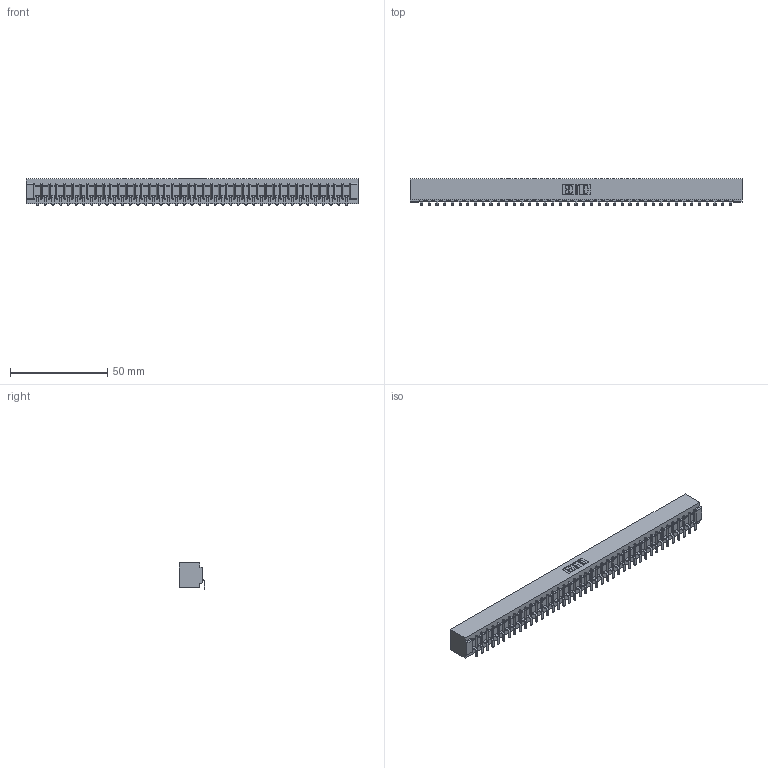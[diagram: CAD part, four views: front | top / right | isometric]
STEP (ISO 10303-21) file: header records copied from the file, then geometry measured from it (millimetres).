
FILE_DESCRIPTION (( 'STEP AP203' ), '1' );
FILE_NAME ('307-041-553-101.STEP', '2019-09-05T11:11:17', ( '' ), ( '' ), 'SwSTEP 2.0', 'SolidWorks 2016', '' );
FILE_SCHEMA (( 'CONFIG_CONTROL_DESIGN' ));
Length unit declared in the file: inch
Products named in the file (3): 307-290-002_553; 307-041-553-101; 307 Part_No Mounting Lugs
Assembly tree (42 placements, depth 2):
  307-041-553-101
    307 Part_No Mounting Lugs
    307-290-002_553  x41
Bounding box: 170.33 x 13.32 x 13.5 mm (x, y, z)
Volume: 18777.8 mm3; surface area: 23931.3 mm2
Topology: 42 solids, 42 shells, 3350 faces, 10303 edges, 6754 vertices
Faces by surface type: plane 1993, cylinder 1273, sphere 84
Entity records: 35848 total; most frequent: CARTESIAN_POINT 6048, ORIENTED_EDGE 6038, DIRECTION 5875, EDGE_CURVE 3019, VECTOR 2313, LINE 2313, VERTEX_POINT 1954, AXIS2_PLACEMENT_3D 1781
